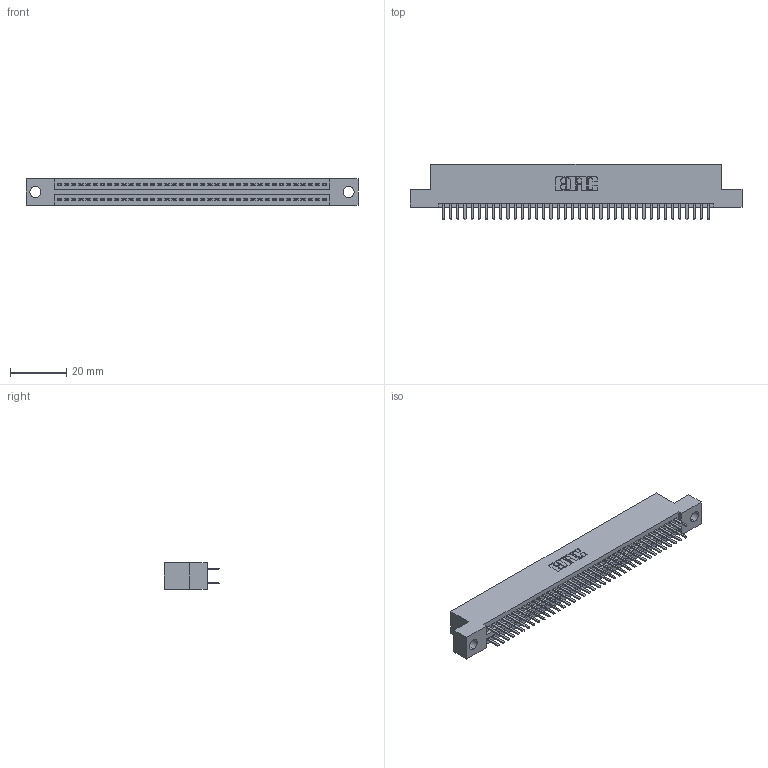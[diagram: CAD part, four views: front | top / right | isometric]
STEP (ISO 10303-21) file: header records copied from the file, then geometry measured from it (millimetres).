
FILE_DESCRIPTION (( 'STEP AP203' ), '1' );
FILE_NAME ('395-076-520-204.STEP', '2018-11-27T20:24:25', ( '' ), ( '' ), 'SwSTEP 2.0', 'SolidWorks 2016', '' );
FILE_SCHEMA (( 'CONFIG_CONTROL_DESIGN' ));
Length unit declared in the file: inch
Products named in the file (3): 345 Part_Flush Mounting Lugs - 0.156 Dia-TH; 395-076-520-204; 345-292-001_345-293-120
Assembly tree (77 placements, depth 2):
  395-076-520-204
    345 Part_Flush Mounting Lugs - 0.156 Dia-TH
    345-292-001_345-293-120  x76
Bounding box: 117.73 x 19.68 x 9.4 mm (x, y, z)
Volume: 11277.9 mm3; surface area: 16337.3 mm2
Topology: 77 solids, 77 shells, 4230 faces, 12273 edges, 7978 vertices
Faces by surface type: plane 2740, cylinder 1490
Entity records: 30471 total; most frequent: CARTESIAN_POINT 5124, ORIENTED_EDGE 5046, DIRECTION 4511, EDGE_CURVE 2523, VECTOR 2235, LINE 2235, VERTEX_POINT 1678, AXIS2_PLACEMENT_3D 1138
